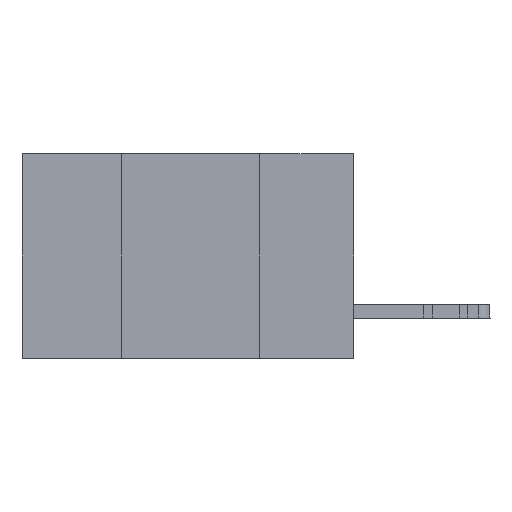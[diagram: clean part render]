
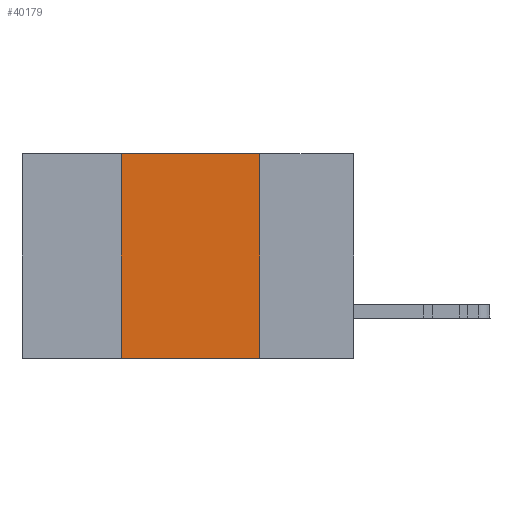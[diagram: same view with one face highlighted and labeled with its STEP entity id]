
A CAD part, left-side view. The second image highlights one B-rep face of the part: STEP entity #40179.
In plain terms, the highlighted planar face has unit normal (-1, 0, 0).
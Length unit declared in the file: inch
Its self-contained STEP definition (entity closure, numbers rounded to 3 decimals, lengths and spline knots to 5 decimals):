
#2236 = FACE_OUTER_BOUND ( 'NONE', #23935, .T. ) ;
#3647 = VERTEX_POINT ( 'NONE', #16977 ) ;
#4446 = AXIS2_PLACEMENT_3D ( 'NONE', #42963, #12483, #29830 ) ;
#7771 = DIRECTION ( 'NONE',  ( 0., -1., 0. ) ) ;
#12483 = DIRECTION ( 'NONE',  ( 1., 0., 0. ) ) ;
#13814 = CARTESIAN_POINT ( 'NONE',  ( 0., 0.17, 0. ) ) ;
#14899 = LINE ( 'NONE', #31798, #43269 ) ;
#15032 = VECTOR ( 'NONE', #43414, 39.37008 ) ;
#16264 = PLANE ( 'NONE',  #4446 ) ;
#16288 = CARTESIAN_POINT ( 'NONE',  ( 0., 0.17, -0.37 ) ) ;
#16586 = EDGE_CURVE ( 'NONE', #22204, #21484, #23950, .T. ) ;
#16977 = CARTESIAN_POINT ( 'NONE',  ( 0., 0.17, 0. ) ) ;
#18205 = ORIENTED_EDGE ( 'NONE', *, *, #22722, .F. ) ;
#18377 = ORIENTED_EDGE ( 'NONE', *, *, #16586, .T. ) ;
#18904 = VERTEX_POINT ( 'NONE', #30712 ) ;
#20635 = ORIENTED_EDGE ( 'NONE', *, *, #27989, .F. ) ;
#21484 = VERTEX_POINT ( 'NONE', #16288 ) ;
#22204 = VERTEX_POINT ( 'NONE', #31095 ) ;
#22722 = EDGE_CURVE ( 'NONE', #22204, #18904, #35864, .T. ) ;
#23935 = EDGE_LOOP ( 'NONE', ( #20635, #25845, #18205, #18377 ) ) ;
#23950 = LINE ( 'NONE', #38386, #33100 ) ;
#25845 = ORIENTED_EDGE ( 'NONE', *, *, #28069, .F. ) ;
#27392 = DIRECTION ( 'NONE',  ( 0., 0., -1. ) ) ;
#27673 = VECTOR ( 'NONE', #27392, 39.37008 ) ;
#27989 = EDGE_CURVE ( 'NONE', #3647, #21484, #30496, .T. ) ;
#28069 = EDGE_CURVE ( 'NONE', #18904, #3647, #14899, .T. ) ;
#29428 = CARTESIAN_POINT ( 'NONE',  ( 0., 0.42, 0. ) ) ;
#29830 = DIRECTION ( 'NONE',  ( 0., 0., -1. ) ) ;
#30496 = LINE ( 'NONE', #13814, #27673 ) ;
#30712 = CARTESIAN_POINT ( 'NONE',  ( 0., 0.42, 0. ) ) ;
#31095 = CARTESIAN_POINT ( 'NONE',  ( 0., 0.42, -0.37 ) ) ;
#31261 = DIRECTION ( 'NONE',  ( 0., -1., 0. ) ) ;
#31798 = CARTESIAN_POINT ( 'NONE',  ( 0., 0.6, 0. ) ) ;
#33100 = VECTOR ( 'NONE', #31261, 39.37008 ) ;
#35864 = LINE ( 'NONE', #29428, #15032 ) ;
#38386 = CARTESIAN_POINT ( 'NONE',  ( 0., 0.6, -0.37 ) ) ;
#40179 = ADVANCED_FACE ( 'NONE', ( #2236 ), #16264, .F. ) ;
#42963 = CARTESIAN_POINT ( 'NONE',  ( 0., 0.6, 0. ) ) ;
#43269 = VECTOR ( 'NONE', #7771, 39.37008 ) ;
#43414 = DIRECTION ( 'NONE',  ( 0., 0., 1. ) ) ;
